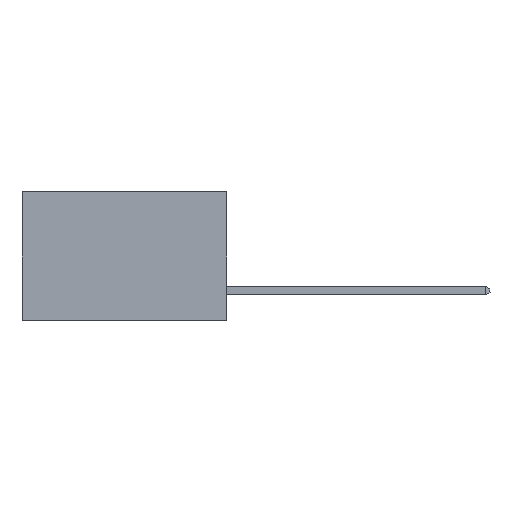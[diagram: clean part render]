
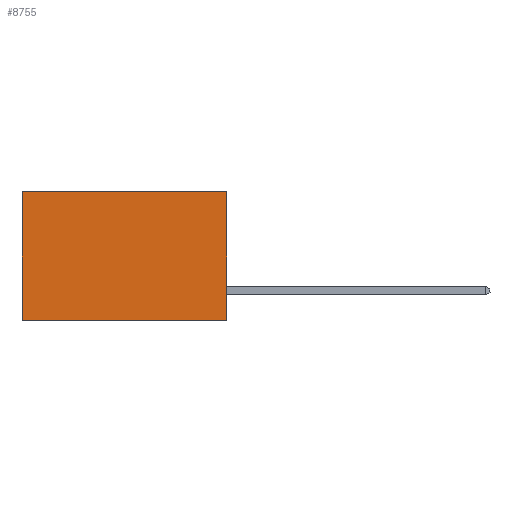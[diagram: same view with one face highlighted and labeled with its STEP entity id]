
A CAD part, left-side view. The second image highlights one B-rep face of the part: STEP entity #8755.
In plain terms, the highlighted planar face has unit normal (-1, 0, 0).
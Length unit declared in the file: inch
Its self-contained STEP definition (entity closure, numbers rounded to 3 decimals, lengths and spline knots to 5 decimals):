
#674 = EDGE_CURVE ( 'NONE', #4501, #4486, #5872, .T. ) ;
#711 = VERTEX_POINT ( 'NONE', #2543 ) ;
#1508 = VECTOR ( 'NONE', #8885, 39.37008 ) ;
#1558 = EDGE_CURVE ( 'NONE', #711, #3598, #5466, .T. ) ;
#1713 = EDGE_CURVE ( 'NONE', #4501, #711, #8385, .T. ) ;
#1820 = EDGE_CURVE ( 'NONE', #4486, #3598, #8776, .T. ) ;
#1946 = VECTOR ( 'NONE', #6741, 39.37008 ) ;
#2392 = CARTESIAN_POINT ( 'NONE',  ( 0.277, 0.59, -0.37 ) ) ;
#2543 = CARTESIAN_POINT ( 'NONE',  ( 0.277, 0., -0.37 ) ) ;
#3167 = VECTOR ( 'NONE', #8811, 39.37008 ) ;
#3590 = VECTOR ( 'NONE', #9723, 39.37008 ) ;
#3598 = VERTEX_POINT ( 'NONE', #9226 ) ;
#4102 = PLANE ( 'NONE',  #8473 ) ;
#4486 = VERTEX_POINT ( 'NONE', #10117 ) ;
#4501 = VERTEX_POINT ( 'NONE', #10598 ) ;
#4715 = FACE_OUTER_BOUND ( 'NONE', #10475, .T. ) ;
#4959 = DIRECTION ( 'NONE',  ( 0., 0., -1. ) ) ;
#5466 = LINE ( 'NONE', #6028, #3167 ) ;
#5546 = CARTESIAN_POINT ( 'NONE',  ( 0.277, 0., -0.37 ) ) ;
#5872 = LINE ( 'NONE', #9865, #3590 ) ;
#6028 = CARTESIAN_POINT ( 'NONE',  ( 0.277, 0., -0.37 ) ) ;
#6611 = CARTESIAN_POINT ( 'NONE',  ( 0.277, 0., -0.37 ) ) ;
#6741 = DIRECTION ( 'NONE',  ( 0., 0., -1. ) ) ;
#8385 = LINE ( 'NONE', #5546, #1508 ) ;
#8473 = AXIS2_PLACEMENT_3D ( 'NONE', #6611, #10017, #4959 ) ;
#8755 = ADVANCED_FACE ( 'NONE', ( #4715 ), #4102, .F. ) ;
#8776 = LINE ( 'NONE', #2392, #1946 ) ;
#8811 = DIRECTION ( 'NONE',  ( 0., 1., 0. ) ) ;
#8885 = DIRECTION ( 'NONE',  ( 0., 0., -1. ) ) ;
#9226 = CARTESIAN_POINT ( 'NONE',  ( 0.277, 0.59, -0.37 ) ) ;
#9723 = DIRECTION ( 'NONE',  ( 0., 1., 0. ) ) ;
#9865 = CARTESIAN_POINT ( 'NONE',  ( 0.277, 0., 0. ) ) ;
#10017 = DIRECTION ( 'NONE',  ( 1., 0., 0. ) ) ;
#10044 = ORIENTED_EDGE ( 'NONE', *, *, #1713, .F. ) ;
#10065 = ORIENTED_EDGE ( 'NONE', *, *, #674, .T. ) ;
#10117 = CARTESIAN_POINT ( 'NONE',  ( 0.277, 0.59, 0. ) ) ;
#10391 = ORIENTED_EDGE ( 'NONE', *, *, #1558, .F. ) ;
#10475 = EDGE_LOOP ( 'NONE', ( #10557, #10391, #10044, #10065 ) ) ;
#10557 = ORIENTED_EDGE ( 'NONE', *, *, #1820, .T. ) ;
#10598 = CARTESIAN_POINT ( 'NONE',  ( 0.277, 0., 0. ) ) ;
